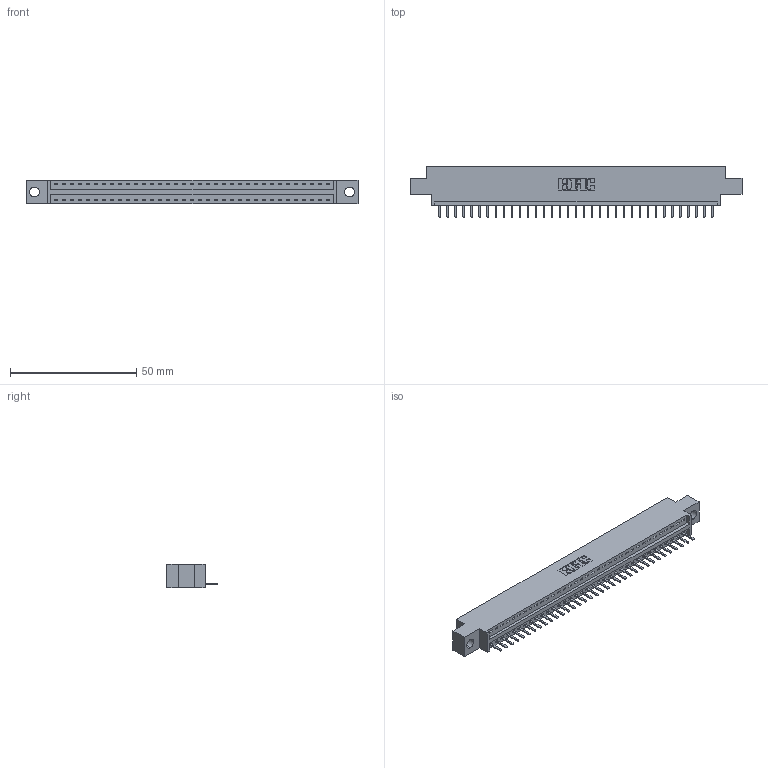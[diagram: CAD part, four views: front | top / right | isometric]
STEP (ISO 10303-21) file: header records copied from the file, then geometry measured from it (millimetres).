
FILE_DESCRIPTION (( 'STEP AP203' ), '1' );
FILE_NAME ('396-035-520-604.STEP', '2018-09-06T02:11:21', ( '' ), ( '' ), 'SwSTEP 2.0', 'SolidWorks 2016', '' );
FILE_SCHEMA (( 'CONFIG_CONTROL_DESIGN' ));
Length unit declared in the file: inch
Products named in the file (3): 396-035-520-604; 346 Part_0.170 Offset - 0.156 Dia-TH; 345-292-001_345-293-120
Assembly tree (36 placements, depth 2):
  396-035-520-604
    346 Part_0.170 Offset - 0.156 Dia-TH
    345-292-001_345-293-120  x35
Bounding box: 131.7 x 20.02 x 9.4 mm (x, y, z)
Volume: 12215.1 mm3; surface area: 14821 mm2
Topology: 36 solids, 36 shells, 2296 faces, 6781 edges, 4426 vertices
Faces by surface type: plane 1550, cylinder 746
Entity records: 22913 total; most frequent: CARTESIAN_POINT 3949, ORIENTED_EDGE 3906, DIRECTION 3479, EDGE_CURVE 1953, VECTOR 1677, LINE 1677, VERTEX_POINT 1298, AXIS2_PLACEMENT_3D 901
